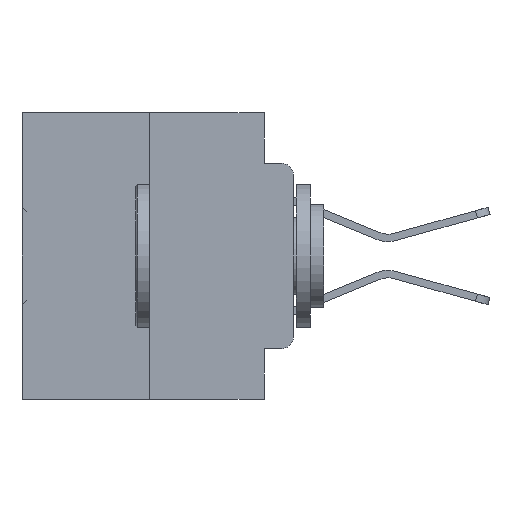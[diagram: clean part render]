
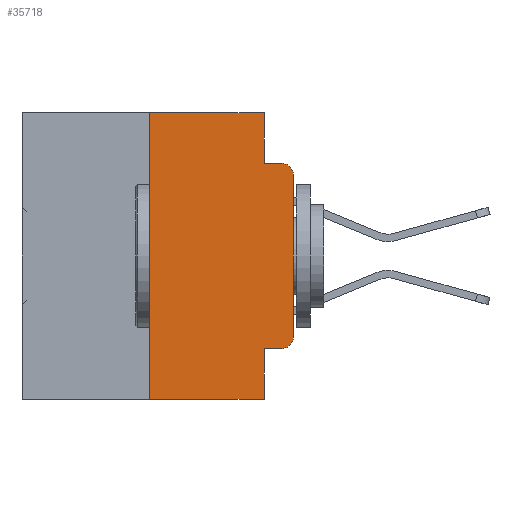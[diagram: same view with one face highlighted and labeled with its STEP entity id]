
A CAD part, left-side view. The second image highlights one B-rep face of the part: STEP entity #35718.
In plain terms, the highlighted planar face has unit normal (-1, 0, 0).
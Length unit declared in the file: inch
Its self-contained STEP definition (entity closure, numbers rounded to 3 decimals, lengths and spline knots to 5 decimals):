
#206 = CARTESIAN_POINT ( 'NONE',  ( 0., 0.473, 0. ) ) ;
#825 = EDGE_CURVE ( 'NONE', #4383, #22485, #20658, .T. ) ;
#1417 = CARTESIAN_POINT ( 'NONE',  ( 0., 0., 0. ) ) ;
#1425 = CARTESIAN_POINT ( 'NONE',  ( 0., 0., -0.3915 ) ) ;
#1840 = ORIENTED_EDGE ( 'NONE', *, *, #22708, .T. ) ;
#3127 = DIRECTION ( 'NONE',  ( 0., -1., 0. ) ) ;
#4383 = VERTEX_POINT ( 'NONE', #1425 ) ;
#4822 = LINE ( 'NONE', #6169, #34254 ) ;
#6169 = CARTESIAN_POINT ( 'NONE',  ( 0., 0.051, 0. ) ) ;
#6681 = DIRECTION ( 'NONE',  ( 0., -1., 0. ) ) ;
#6916 = CARTESIAN_POINT ( 'NONE',  ( 0., 0.02, -0.3915 ) ) ;
#7007 = DIRECTION ( 'NONE',  ( 0., -1., 0. ) ) ;
#7284 = CARTESIAN_POINT ( 'NONE',  ( 0., 0.02, -0.4115 ) ) ;
#7530 = CARTESIAN_POINT ( 'NONE',  ( 0., 0.25, 0. ) ) ;
#8234 = ORIENTED_EDGE ( 'NONE', *, *, #825, .T. ) ;
#8951 = DIRECTION ( 'NONE',  ( 0., 0., 1. ) ) ;
#9296 = LINE ( 'NONE', #17968, #30178 ) ;
#9835 = DIRECTION ( 'NONE',  ( 0., 0., -1. ) ) ;
#9927 = CARTESIAN_POINT ( 'NONE',  ( 0., 0.051, -0.4115 ) ) ;
#10122 = CARTESIAN_POINT ( 'NONE',  ( 0., 0.051, -0.4115 ) ) ;
#10282 = CARTESIAN_POINT ( 'NONE',  ( 0., 0.25, 0. ) ) ;
#10306 = CIRCLE ( 'NONE', #26803, 0.02 ) ;
#10462 = DIRECTION ( 'NONE',  ( -1., 0., 0. ) ) ;
#10549 = VECTOR ( 'NONE', #30303, 39.37008 ) ;
#14378 = AXIS2_PLACEMENT_3D ( 'NONE', #27430, #10462, #21503 ) ;
#14533 = VERTEX_POINT ( 'NONE', #10282 ) ;
#15070 = LINE ( 'NONE', #206, #35849 ) ;
#15874 = ORIENTED_EDGE ( 'NONE', *, *, #36003, .T. ) ;
#16336 = ORIENTED_EDGE ( 'NONE', *, *, #24581, .F. ) ;
#17465 = LINE ( 'NONE', #18433, #24058 ) ;
#17543 = EDGE_CURVE ( 'NONE', #24060, #28898, #17465, .T. ) ;
#17608 = VERTEX_POINT ( 'NONE', #7284 ) ;
#17722 = DIRECTION ( 'NONE',  ( 0., 0., -1. ) ) ;
#17968 = CARTESIAN_POINT ( 'NONE',  ( 0., 0.051, -0.0885 ) ) ;
#18433 = CARTESIAN_POINT ( 'NONE',  ( 0., 0.473, -0.5 ) ) ;
#18789 = CARTESIAN_POINT ( 'NONE',  ( 0., 0.02, -0.0885 ) ) ;
#19113 = VERTEX_POINT ( 'NONE', #18789 ) ;
#19607 = EDGE_LOOP ( 'NONE', ( #8234, #15874, #25107, #25994, #20282, #35338, #36226, #16336, #1840, #33148 ) ) ;
#19710 = VERTEX_POINT ( 'NONE', #21363 ) ;
#19759 = VECTOR ( 'NONE', #8951, 39.37008 ) ;
#20046 = DIRECTION ( 'NONE',  ( 0., 0., -1. ) ) ;
#20256 = CARTESIAN_POINT ( 'NONE',  ( 0., 0., -0.1085 ) ) ;
#20282 = ORIENTED_EDGE ( 'NONE', *, *, #33192, .F. ) ;
#20597 = CIRCLE ( 'NONE', #14378, 0.02 ) ;
#20658 = LINE ( 'NONE', #1417, #19759 ) ;
#20762 = AXIS2_PLACEMENT_3D ( 'NONE', #34162, #37006, #20046 ) ;
#20836 = EDGE_CURVE ( 'NONE', #17608, #4383, #10306, .T. ) ;
#21010 = CARTESIAN_POINT ( 'NONE',  ( 0., 0.051, -0.0885 ) ) ;
#21071 = FACE_OUTER_BOUND ( 'NONE', #19607, .T. ) ;
#21241 = CARTESIAN_POINT ( 'NONE',  ( 0., 0.051, -0.5 ) ) ;
#21363 = CARTESIAN_POINT ( 'NONE',  ( 0., 0.051, 0. ) ) ;
#21503 = DIRECTION ( 'NONE',  ( 0., 0., -1. ) ) ;
#22216 = LINE ( 'NONE', #9927, #27945 ) ;
#22485 = VERTEX_POINT ( 'NONE', #20256 ) ;
#22621 = VERTEX_POINT ( 'NONE', #21010 ) ;
#22708 = EDGE_CURVE ( 'NONE', #35422, #17608, #22216, .T. ) ;
#22799 = VECTOR ( 'NONE', #34100, 39.37008 ) ;
#24058 = VECTOR ( 'NONE', #32563, 39.37008 ) ;
#24060 = VERTEX_POINT ( 'NONE', #24816 ) ;
#24581 = EDGE_CURVE ( 'NONE', #35422, #28898, #30361, .T. ) ;
#24816 = CARTESIAN_POINT ( 'NONE',  ( 0., 0.25, -0.5 ) ) ;
#25107 = ORIENTED_EDGE ( 'NONE', *, *, #32206, .F. ) ;
#25592 = LINE ( 'NONE', #7530, #10549 ) ;
#25994 = ORIENTED_EDGE ( 'NONE', *, *, #30325, .F. ) ;
#26803 = AXIS2_PLACEMENT_3D ( 'NONE', #6916, #26824, #9835 ) ;
#26824 = DIRECTION ( 'NONE',  ( -1., 0., 0. ) ) ;
#27430 = CARTESIAN_POINT ( 'NONE',  ( 0., 0.02, -0.1085 ) ) ;
#27945 = VECTOR ( 'NONE', #7007, 39.37008 ) ;
#28399 = EDGE_CURVE ( 'NONE', #24060, #14533, #25592, .T. ) ;
#28451 = PLANE ( 'NONE',  #20762 ) ;
#28898 = VERTEX_POINT ( 'NONE', #21241 ) ;
#30178 = VECTOR ( 'NONE', #6681, 39.37008 ) ;
#30303 = DIRECTION ( 'NONE',  ( 0., 0., 1. ) ) ;
#30325 = EDGE_CURVE ( 'NONE', #19710, #22621, #4822, .T. ) ;
#30361 = LINE ( 'NONE', #36819, #22799 ) ;
#32206 = EDGE_CURVE ( 'NONE', #22621, #19113, #9296, .T. ) ;
#32563 = DIRECTION ( 'NONE',  ( 0., -1., 0. ) ) ;
#33148 = ORIENTED_EDGE ( 'NONE', *, *, #20836, .T. ) ;
#33192 = EDGE_CURVE ( 'NONE', #14533, #19710, #15070, .T. ) ;
#34100 = DIRECTION ( 'NONE',  ( 0., 0., -1. ) ) ;
#34162 = CARTESIAN_POINT ( 'NONE',  ( 0., 0.473, 0. ) ) ;
#34254 = VECTOR ( 'NONE', #17722, 39.37008 ) ;
#35338 = ORIENTED_EDGE ( 'NONE', *, *, #28399, .F. ) ;
#35422 = VERTEX_POINT ( 'NONE', #10122 ) ;
#35718 = ADVANCED_FACE ( 'NONE', ( #21071 ), #28451, .F. ) ;
#35849 = VECTOR ( 'NONE', #3127, 39.37008 ) ;
#36003 = EDGE_CURVE ( 'NONE', #22485, #19113, #20597, .T. ) ;
#36226 = ORIENTED_EDGE ( 'NONE', *, *, #17543, .T. ) ;
#36819 = CARTESIAN_POINT ( 'NONE',  ( 0., 0.051, 0. ) ) ;
#37006 = DIRECTION ( 'NONE',  ( 1., 0., 0. ) ) ;
